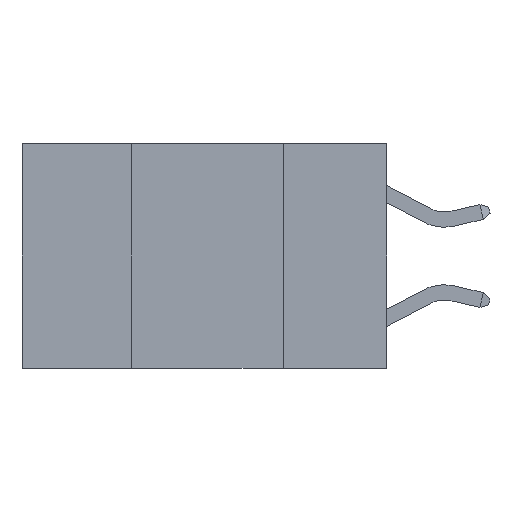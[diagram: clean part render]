
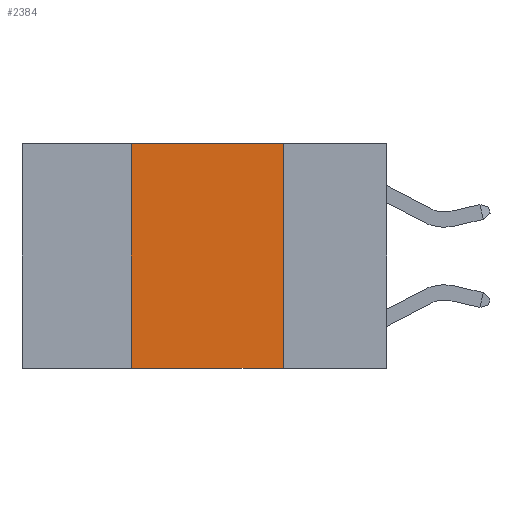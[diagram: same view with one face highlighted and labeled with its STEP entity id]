
A CAD part, left-side view. The second image highlights one B-rep face of the part: STEP entity #2384.
In plain terms, the highlighted planar face has unit normal (-1, 0, 0).
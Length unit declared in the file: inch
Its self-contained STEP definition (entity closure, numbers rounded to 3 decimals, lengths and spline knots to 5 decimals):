
#74 = DIRECTION ( 'NONE',  ( 0., 0., 1. ) ) ;
#162 = DIRECTION ( 'NONE',  ( 0., 0., -1. ) ) ;
#256 = DIRECTION ( 'NONE',  ( 0., 0., -1. ) ) ;
#888 = ORIENTED_EDGE ( 'NONE', *, *, #5973, .F. ) ;
#1154 = DIRECTION ( 'NONE',  ( 0., -1., 0. ) ) ;
#1480 = LINE ( 'NONE', #6877, #4811 ) ;
#1689 = DIRECTION ( 'NONE',  ( 1., 0., 0. ) ) ;
#2384 = ADVANCED_FACE ( 'NONE', ( #8686 ), #2461, .F. ) ;
#2461 = PLANE ( 'NONE',  #7907 ) ;
#2734 = VERTEX_POINT ( 'NONE', #6743 ) ;
#3490 = VECTOR ( 'NONE', #1154, 39.37008 ) ;
#3671 = CARTESIAN_POINT ( 'NONE',  ( 0., 0.42, -0.37 ) ) ;
#3719 = ORIENTED_EDGE ( 'NONE', *, *, #9352, .F. ) ;
#3979 = VECTOR ( 'NONE', #74, 39.37008 ) ;
#4184 = CARTESIAN_POINT ( 'NONE',  ( 0., 0.6, 0. ) ) ;
#4473 = CARTESIAN_POINT ( 'NONE',  ( 0., 0.17, -0.37 ) ) ;
#4811 = VECTOR ( 'NONE', #10018, 39.37008 ) ;
#4840 = CARTESIAN_POINT ( 'NONE',  ( 0., 0.17, 0. ) ) ;
#5098 = VERTEX_POINT ( 'NONE', #4473 ) ;
#5676 = LINE ( 'NONE', #4840, #7287 ) ;
#5973 = EDGE_CURVE ( 'NONE', #8050, #2734, #8376, .T. ) ;
#6743 = CARTESIAN_POINT ( 'NONE',  ( 0., 0.17, 0. ) ) ;
#6749 = EDGE_CURVE ( 'NONE', #2734, #5098, #5676, .T. ) ;
#6783 = ORIENTED_EDGE ( 'NONE', *, *, #6749, .F. ) ;
#6877 = CARTESIAN_POINT ( 'NONE',  ( 0., 0.6, -0.37 ) ) ;
#7287 = VECTOR ( 'NONE', #162, 39.37008 ) ;
#7368 = ORIENTED_EDGE ( 'NONE', *, *, #9225, .T. ) ;
#7797 = CARTESIAN_POINT ( 'NONE',  ( 0., 0.42, 0. ) ) ;
#7849 = LINE ( 'NONE', #7797, #3979 ) ;
#7907 = AXIS2_PLACEMENT_3D ( 'NONE', #8732, #1689, #256 ) ;
#8050 = VERTEX_POINT ( 'NONE', #8715 ) ;
#8344 = EDGE_LOOP ( 'NONE', ( #6783, #888, #3719, #7368 ) ) ;
#8376 = LINE ( 'NONE', #4184, #3490 ) ;
#8686 = FACE_OUTER_BOUND ( 'NONE', #8344, .T. ) ;
#8715 = CARTESIAN_POINT ( 'NONE',  ( 0., 0.42, 0. ) ) ;
#8732 = CARTESIAN_POINT ( 'NONE',  ( 0., 0.6, 0. ) ) ;
#9182 = VERTEX_POINT ( 'NONE', #3671 ) ;
#9225 = EDGE_CURVE ( 'NONE', #9182, #5098, #1480, .T. ) ;
#9352 = EDGE_CURVE ( 'NONE', #9182, #8050, #7849, .T. ) ;
#10018 = DIRECTION ( 'NONE',  ( 0., -1., 0. ) ) ;
